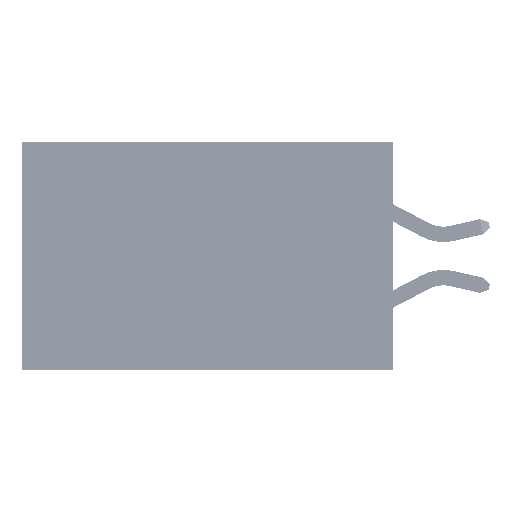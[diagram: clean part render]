
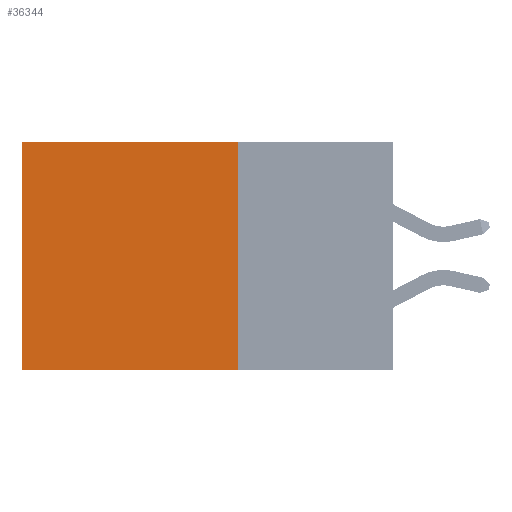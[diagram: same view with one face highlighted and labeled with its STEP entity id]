
A CAD part, left-side view. The second image highlights one B-rep face of the part: STEP entity #36344.
In plain terms, the highlighted planar face has unit normal (-1, 0, 0).
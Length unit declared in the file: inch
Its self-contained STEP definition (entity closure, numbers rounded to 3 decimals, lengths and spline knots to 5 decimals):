
#581 = LINE ( 'NONE', #9922, #38089 ) ;
#3392 = EDGE_LOOP ( 'NONE', ( #8408, #29254, #48436, #46015 ) ) ;
#4203 = CARTESIAN_POINT ( 'NONE',  ( 0.2875, 0.6, -0.37 ) ) ;
#4711 = CARTESIAN_POINT ( 'NONE',  ( 0.2875, 0.25, 0. ) ) ;
#4874 = CARTESIAN_POINT ( 'NONE',  ( 0.2875, 0.25, -0.37 ) ) ;
#5446 = VERTEX_POINT ( 'NONE', #14038 ) ;
#6481 = PLANE ( 'NONE',  #49296 ) ;
#6571 = LINE ( 'NONE', #4711, #36262 ) ;
#8408 = ORIENTED_EDGE ( 'NONE', *, *, #11432, .T. ) ;
#9922 = CARTESIAN_POINT ( 'NONE',  ( 0.2875, 0.6, 0. ) ) ;
#10151 = EDGE_CURVE ( 'NONE', #46503, #18199, #35852, .T. ) ;
#10374 = CARTESIAN_POINT ( 'NONE',  ( 0.2875, 0.25, 0. ) ) ;
#11432 = EDGE_CURVE ( 'NONE', #5446, #31798, #581, .T. ) ;
#14038 = CARTESIAN_POINT ( 'NONE',  ( 0.2875, 0.6, 0. ) ) ;
#16861 = FACE_OUTER_BOUND ( 'NONE', #3392, .T. ) ;
#18049 = CARTESIAN_POINT ( 'NONE',  ( 0.2875, 0.25, 0. ) ) ;
#18199 = VERTEX_POINT ( 'NONE', #4874 ) ;
#21367 = CARTESIAN_POINT ( 'NONE',  ( 0.2875, 0.25, -0.37 ) ) ;
#21793 = DIRECTION ( 'NONE',  ( 0., 0., -1. ) ) ;
#22472 = EDGE_CURVE ( 'NONE', #18199, #31798, #42747, .T. ) ;
#23117 = VECTOR ( 'NONE', #21793, 39.37008 ) ;
#25323 = DIRECTION ( 'NONE',  ( 0., 0., -1. ) ) ;
#27722 = DIRECTION ( 'NONE',  ( 0., 1., 0. ) ) ;
#28566 = EDGE_CURVE ( 'NONE', #46503, #5446, #6571, .T. ) ;
#29254 = ORIENTED_EDGE ( 'NONE', *, *, #22472, .F. ) ;
#31798 = VERTEX_POINT ( 'NONE', #4203 ) ;
#32708 = DIRECTION ( 'NONE',  ( 0., 1., 0. ) ) ;
#35852 = LINE ( 'NONE', #18049, #23117 ) ;
#36262 = VECTOR ( 'NONE', #27722, 39.37008 ) ;
#36344 = ADVANCED_FACE ( 'NONE', ( #16861 ), #6481, .F. ) ;
#38089 = VECTOR ( 'NONE', #45284, 39.37008 ) ;
#39697 = VECTOR ( 'NONE', #32708, 39.37008 ) ;
#42747 = LINE ( 'NONE', #21367, #39697 ) ;
#44258 = CARTESIAN_POINT ( 'NONE',  ( 0.2875, 0.25, 0. ) ) ;
#44914 = DIRECTION ( 'NONE',  ( 1., 0., 0. ) ) ;
#45284 = DIRECTION ( 'NONE',  ( 0., 0., -1. ) ) ;
#46015 = ORIENTED_EDGE ( 'NONE', *, *, #28566, .T. ) ;
#46503 = VERTEX_POINT ( 'NONE', #44258 ) ;
#48436 = ORIENTED_EDGE ( 'NONE', *, *, #10151, .F. ) ;
#49296 = AXIS2_PLACEMENT_3D ( 'NONE', #10374, #44914, #25323 ) ;
